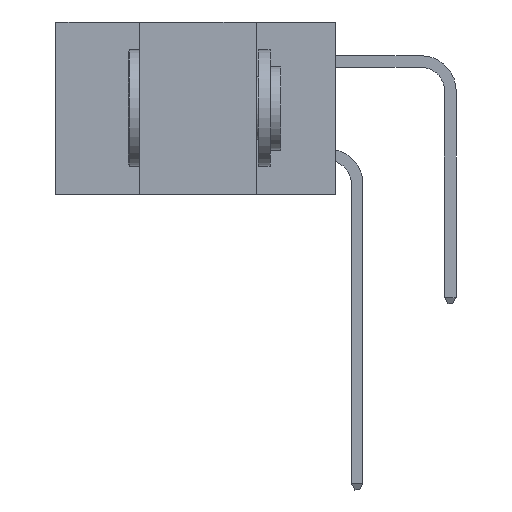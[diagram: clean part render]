
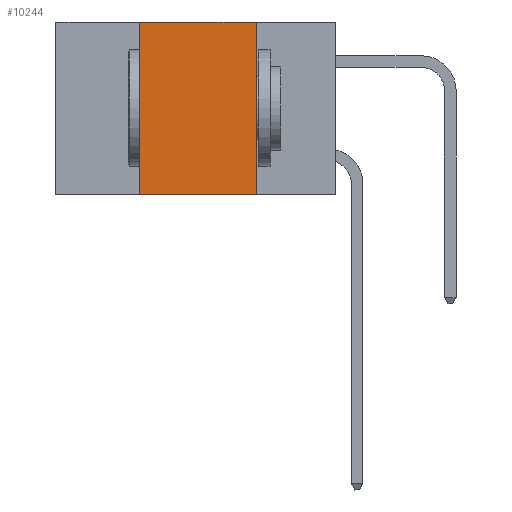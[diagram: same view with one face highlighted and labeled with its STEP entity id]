
A CAD part, left-side view. The second image highlights one B-rep face of the part: STEP entity #10244.
In plain terms, the highlighted planar face has unit normal (-1, 0, 0).
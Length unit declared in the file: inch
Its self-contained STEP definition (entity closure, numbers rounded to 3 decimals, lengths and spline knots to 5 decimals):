
#490 = EDGE_CURVE ( 'NONE', #2181, #21083, #9401, .T. ) ;
#2181 = VERTEX_POINT ( 'NONE', #8082 ) ;
#2408 = ORIENTED_EDGE ( 'NONE', *, *, #15897, .F. ) ;
#2786 = CARTESIAN_POINT ( 'NONE',  ( 0., 0.6, 0. ) ) ;
#3071 = VECTOR ( 'NONE', #5248, 39.37008 ) ;
#3267 = CARTESIAN_POINT ( 'NONE',  ( 0., 0.42, 0. ) ) ;
#5085 = EDGE_LOOP ( 'NONE', ( #17349, #2408, #28995, #11661 ) ) ;
#5187 = DIRECTION ( 'NONE',  ( 0., -1., 0. ) ) ;
#5248 = DIRECTION ( 'NONE',  ( 0., 0., -1. ) ) ;
#5448 = CARTESIAN_POINT ( 'NONE',  ( 0., 0.17, 0. ) ) ;
#5513 = PLANE ( 'NONE',  #22006 ) ;
#8082 = CARTESIAN_POINT ( 'NONE',  ( 0., 0.17, 0. ) ) ;
#9401 = LINE ( 'NONE', #5448, #3071 ) ;
#9967 = VECTOR ( 'NONE', #5187, 39.37008 ) ;
#9968 = EDGE_CURVE ( 'NONE', #21355, #16749, #15201, .T. ) ;
#10244 = ADVANCED_FACE ( 'NONE', ( #19753 ), #5513, .F. ) ;
#10299 = CARTESIAN_POINT ( 'NONE',  ( 0., 0.6, 0. ) ) ;
#11661 = ORIENTED_EDGE ( 'NONE', *, *, #29106, .T. ) ;
#12710 = DIRECTION ( 'NONE',  ( 1., 0., 0. ) ) ;
#14817 = VECTOR ( 'NONE', #23665, 39.37008 ) ;
#15201 = LINE ( 'NONE', #28332, #27112 ) ;
#15414 = CARTESIAN_POINT ( 'NONE',  ( 0., 0.17, -0.37 ) ) ;
#15579 = LINE ( 'NONE', #30727, #14817 ) ;
#15897 = EDGE_CURVE ( 'NONE', #16749, #2181, #28945, .T. ) ;
#16454 = CARTESIAN_POINT ( 'NONE',  ( 0., 0.42, -0.37 ) ) ;
#16532 = DIRECTION ( 'NONE',  ( 0., 0., 1. ) ) ;
#16749 = VERTEX_POINT ( 'NONE', #3267 ) ;
#17349 = ORIENTED_EDGE ( 'NONE', *, *, #490, .F. ) ;
#19753 = FACE_OUTER_BOUND ( 'NONE', #5085, .T. ) ;
#21083 = VERTEX_POINT ( 'NONE', #15414 ) ;
#21355 = VERTEX_POINT ( 'NONE', #16454 ) ;
#22006 = AXIS2_PLACEMENT_3D ( 'NONE', #10299, #12710, #29331 ) ;
#23665 = DIRECTION ( 'NONE',  ( 0., -1., 0. ) ) ;
#27112 = VECTOR ( 'NONE', #16532, 39.37008 ) ;
#28332 = CARTESIAN_POINT ( 'NONE',  ( 0., 0.42, 0. ) ) ;
#28945 = LINE ( 'NONE', #2786, #9967 ) ;
#28995 = ORIENTED_EDGE ( 'NONE', *, *, #9968, .F. ) ;
#29106 = EDGE_CURVE ( 'NONE', #21355, #21083, #15579, .T. ) ;
#29331 = DIRECTION ( 'NONE',  ( 0., 0., -1. ) ) ;
#30727 = CARTESIAN_POINT ( 'NONE',  ( 0., 0.6, -0.37 ) ) ;
